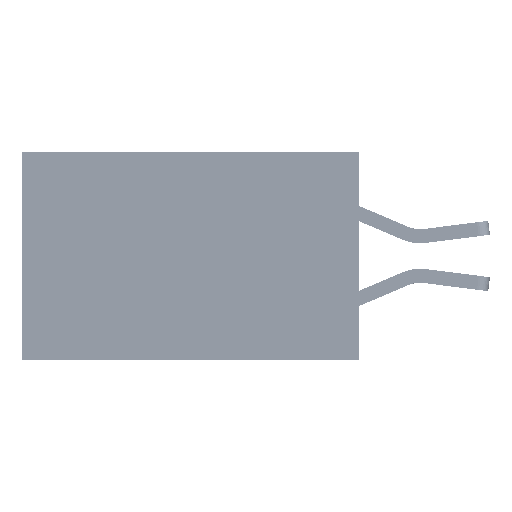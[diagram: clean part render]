
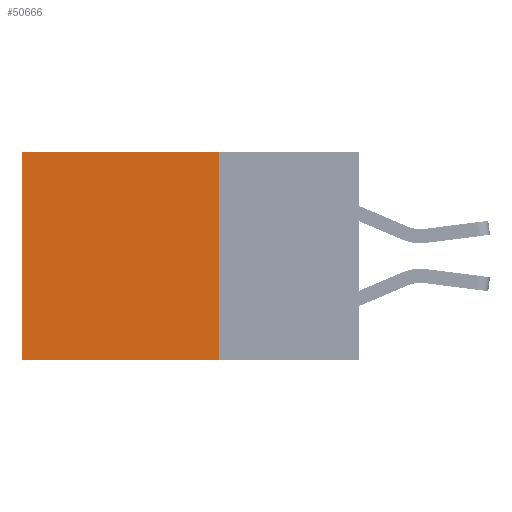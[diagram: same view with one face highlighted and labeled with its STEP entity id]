
A CAD part, left-side view. The second image highlights one B-rep face of the part: STEP entity #50666.
In plain terms, the highlighted planar face has unit normal (-1, 0, 0).
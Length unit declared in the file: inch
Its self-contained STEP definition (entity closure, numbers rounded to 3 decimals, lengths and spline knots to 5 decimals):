
#2439 = DIRECTION ( 'NONE',  ( 0., 1., 0. ) ) ;
#2934 = VERTEX_POINT ( 'NONE', #36489 ) ;
#4252 = PLANE ( 'NONE',  #20569 ) ;
#6289 = ORIENTED_EDGE ( 'NONE', *, *, #38547, .F. ) ;
#7000 = EDGE_CURVE ( 'NONE', #9053, #46669, #50416, .T. ) ;
#7486 = CARTESIAN_POINT ( 'NONE',  ( 0.2875, 0.6, 0. ) ) ;
#9053 = VERTEX_POINT ( 'NONE', #44993 ) ;
#11280 = VERTEX_POINT ( 'NONE', #21835 ) ;
#11418 = EDGE_CURVE ( 'NONE', #9053, #11280, #37253, .T. ) ;
#12207 = DIRECTION ( 'NONE',  ( 0., 0., -1. ) ) ;
#14540 = DIRECTION ( 'NONE',  ( 0., 0., -1. ) ) ;
#15345 = VECTOR ( 'NONE', #40191, 39.37008 ) ;
#16545 = CARTESIAN_POINT ( 'NONE',  ( 0.2875, 0.6, 0. ) ) ;
#19314 = EDGE_LOOP ( 'NONE', ( #39489, #6289, #34540, #32308 ) ) ;
#20569 = AXIS2_PLACEMENT_3D ( 'NONE', #31878, #35790, #12207 ) ;
#21835 = CARTESIAN_POINT ( 'NONE',  ( 0.2875, 0.25, -0.37 ) ) ;
#23149 = DIRECTION ( 'NONE',  ( 0., 1., 0. ) ) ;
#25642 = VECTOR ( 'NONE', #14540, 39.37008 ) ;
#25891 = LINE ( 'NONE', #16545, #15345 ) ;
#31878 = CARTESIAN_POINT ( 'NONE',  ( 0.2875, 0.25, 0. ) ) ;
#32308 = ORIENTED_EDGE ( 'NONE', *, *, #7000, .T. ) ;
#34183 = CARTESIAN_POINT ( 'NONE',  ( 0.2875, 0.25, 0. ) ) ;
#34540 = ORIENTED_EDGE ( 'NONE', *, *, #11418, .F. ) ;
#35790 = DIRECTION ( 'NONE',  ( 1., 0., 0. ) ) ;
#36489 = CARTESIAN_POINT ( 'NONE',  ( 0.2875, 0.6, -0.37 ) ) ;
#37253 = LINE ( 'NONE', #34183, #25642 ) ;
#38547 = EDGE_CURVE ( 'NONE', #11280, #2934, #50336, .T. ) ;
#39098 = FACE_OUTER_BOUND ( 'NONE', #19314, .T. ) ;
#39489 = ORIENTED_EDGE ( 'NONE', *, *, #50043, .T. ) ;
#40083 = VECTOR ( 'NONE', #23149, 39.37008 ) ;
#40191 = DIRECTION ( 'NONE',  ( 0., 0., -1. ) ) ;
#44993 = CARTESIAN_POINT ( 'NONE',  ( 0.2875, 0.25, 0. ) ) ;
#46669 = VERTEX_POINT ( 'NONE', #7486 ) ;
#49104 = VECTOR ( 'NONE', #2439, 39.37008 ) ;
#49502 = CARTESIAN_POINT ( 'NONE',  ( 0.2875, 0.25, -0.37 ) ) ;
#50043 = EDGE_CURVE ( 'NONE', #46669, #2934, #25891, .T. ) ;
#50336 = LINE ( 'NONE', #49502, #49104 ) ;
#50416 = LINE ( 'NONE', #50597, #40083 ) ;
#50597 = CARTESIAN_POINT ( 'NONE',  ( 0.2875, 0.25, 0. ) ) ;
#50666 = ADVANCED_FACE ( 'NONE', ( #39098 ), #4252, .F. ) ;
